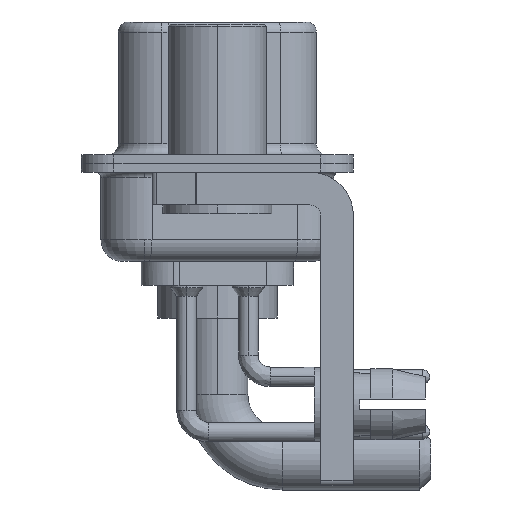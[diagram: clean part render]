
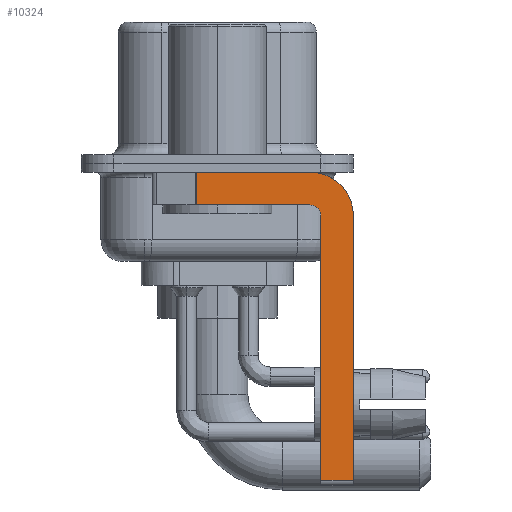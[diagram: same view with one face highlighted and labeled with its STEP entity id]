
A CAD part, left-side view. The second image highlights one B-rep face of the part: STEP entity #10324.
In plain terms, the highlighted planar face has unit normal (-1, 0, 0).
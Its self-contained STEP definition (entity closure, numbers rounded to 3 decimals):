
#198 = CARTESIAN_POINT ( 'NONE',  ( -2.9, 0.978, -0.4 ) ) ;
#561 = VERTEX_POINT ( 'NONE', #11415 ) ;
#742 = CARTESIAN_POINT ( 'NONE',  ( -2.9, -6.25, -2.4 ) ) ;
#893 = ORIENTED_EDGE ( 'NONE', *, *, #22448, .F. ) ;
#1532 = DIRECTION ( 'NONE',  ( 0., 0., -1. ) ) ;
#2229 = CARTESIAN_POINT ( 'NONE',  ( -2.9, -6.25, -14.55 ) ) ;
#2607 = AXIS2_PLACEMENT_3D ( 'NONE', #18476, #2618, #9718 ) ;
#2618 = DIRECTION ( 'NONE',  ( -1., 0., 0. ) ) ;
#2639 = VECTOR ( 'NONE', #4369, 1000. ) ;
#3661 = LINE ( 'NONE', #16160, #8724 ) ;
#3968 = DIRECTION ( 'NONE',  ( 1., 0., 0. ) ) ;
#4296 = VECTOR ( 'NONE', #12155, 1000. ) ;
#4369 = DIRECTION ( 'NONE',  ( 0., 0., 1. ) ) ;
#4706 = CIRCLE ( 'NONE', #19837, 2. ) ;
#4944 = ORIENTED_EDGE ( 'NONE', *, *, #9349, .F. ) ;
#5148 = LINE ( 'NONE', #17402, #20176 ) ;
#5156 = ORIENTED_EDGE ( 'NONE', *, *, #17965, .F. ) ;
#5407 = DIRECTION ( 'NONE',  ( 0., 1., 0. ) ) ;
#5773 = CARTESIAN_POINT ( 'NONE',  ( -2.9, -4.75, -14.55 ) ) ;
#6127 = CARTESIAN_POINT ( 'NONE',  ( -2.9, -4.25, -2.4 ) ) ;
#6393 = VECTOR ( 'NONE', #16126, 1000. ) ;
#6450 = VERTEX_POINT ( 'NONE', #198 ) ;
#7355 = DIRECTION ( 'NONE',  ( 0., 0., -1. ) ) ;
#7446 = CARTESIAN_POINT ( 'NONE',  ( -2.9, -4.75, -14.8 ) ) ;
#7569 = ORIENTED_EDGE ( 'NONE', *, *, #19636, .T. ) ;
#7579 = PLANE ( 'NONE',  #13545 ) ;
#7829 = VERTEX_POINT ( 'NONE', #5773 ) ;
#8724 = VECTOR ( 'NONE', #5407, 1000. ) ;
#9063 = CARTESIAN_POINT ( 'NONE',  ( -2.9, 0.978, -1.9 ) ) ;
#9349 = EDGE_CURVE ( 'NONE', #21765, #10509, #3661, .T. ) ;
#9489 = VERTEX_POINT ( 'NONE', #742 ) ;
#9662 = CIRCLE ( 'NONE', #2607, 0.5 ) ;
#9718 = DIRECTION ( 'NONE',  ( 0., 0., 1. ) ) ;
#9964 = DIRECTION ( 'NONE',  ( 1., 0., 0. ) ) ;
#10172 = ORIENTED_EDGE ( 'NONE', *, *, #18957, .F. ) ;
#10324 = ADVANCED_FACE ( 'NONE', ( #20044 ), #7579, .F. ) ;
#10509 = VERTEX_POINT ( 'NONE', #9063 ) ;
#10630 = CARTESIAN_POINT ( 'NONE',  ( -2.9, -4.75, -2.4 ) ) ;
#11415 = CARTESIAN_POINT ( 'NONE',  ( -2.9, -4.25, -0.4 ) ) ;
#11485 = EDGE_LOOP ( 'NONE', ( #893, #13242, #4944, #5156, #10172, #7569, #13227, #17804 ) ) ;
#11823 = VECTOR ( 'NONE', #7355, 1000. ) ;
#12090 = VERTEX_POINT ( 'NONE', #2229 ) ;
#12155 = DIRECTION ( 'NONE',  ( 0., -1., 0. ) ) ;
#12673 = EDGE_CURVE ( 'NONE', #561, #9489, #4706, .T. ) ;
#12778 = DIRECTION ( 'NONE',  ( 0., 0., -1. ) ) ;
#13111 = CARTESIAN_POINT ( 'NONE',  ( -2.9, -4.25, -2.4 ) ) ;
#13227 = ORIENTED_EDGE ( 'NONE', *, *, #22737, .F. ) ;
#13242 = ORIENTED_EDGE ( 'NONE', *, *, #15079, .T. ) ;
#13545 = AXIS2_PLACEMENT_3D ( 'NONE', #13111, #3968, #12778 ) ;
#13547 = CARTESIAN_POINT ( 'NONE',  ( -2.9, -4.25, -1.9 ) ) ;
#14495 = CARTESIAN_POINT ( 'NONE',  ( -2.9, 0.978, -1.9 ) ) ;
#15079 = EDGE_CURVE ( 'NONE', #6450, #10509, #16120, .T. ) ;
#15266 = CARTESIAN_POINT ( 'NONE',  ( -2.9, 3., -0.4 ) ) ;
#15605 = LINE ( 'NONE', #15266, #4296 ) ;
#16120 = LINE ( 'NONE', #14495, #11823 ) ;
#16126 = DIRECTION ( 'NONE',  ( 0., -1., 0. ) ) ;
#16160 = CARTESIAN_POINT ( 'NONE',  ( -2.9, -4.25, -1.9 ) ) ;
#16244 = LINE ( 'NONE', #19592, #6393 ) ;
#17402 = CARTESIAN_POINT ( 'NONE',  ( -2.9, -6.25, -2.4 ) ) ;
#17804 = ORIENTED_EDGE ( 'NONE', *, *, #12673, .F. ) ;
#17965 = EDGE_CURVE ( 'NONE', #18273, #21765, #9662, .T. ) ;
#18273 = VERTEX_POINT ( 'NONE', #10630 ) ;
#18476 = CARTESIAN_POINT ( 'NONE',  ( -2.9, -4.25, -2.4 ) ) ;
#18957 = EDGE_CURVE ( 'NONE', #7829, #18273, #20215, .T. ) ;
#19592 = CARTESIAN_POINT ( 'NONE',  ( -2.9, -4.25, -14.55 ) ) ;
#19636 = EDGE_CURVE ( 'NONE', #7829, #12090, #16244, .T. ) ;
#19837 = AXIS2_PLACEMENT_3D ( 'NONE', #6127, #9964, #20227 ) ;
#20044 = FACE_OUTER_BOUND ( 'NONE', #11485, .T. ) ;
#20176 = VECTOR ( 'NONE', #1532, 1000. ) ;
#20215 = LINE ( 'NONE', #7446, #2639 ) ;
#20227 = DIRECTION ( 'NONE',  ( 0., 0., -1. ) ) ;
#21765 = VERTEX_POINT ( 'NONE', #13547 ) ;
#22448 = EDGE_CURVE ( 'NONE', #6450, #561, #15605, .T. ) ;
#22737 = EDGE_CURVE ( 'NONE', #9489, #12090, #5148, .T. ) ;
